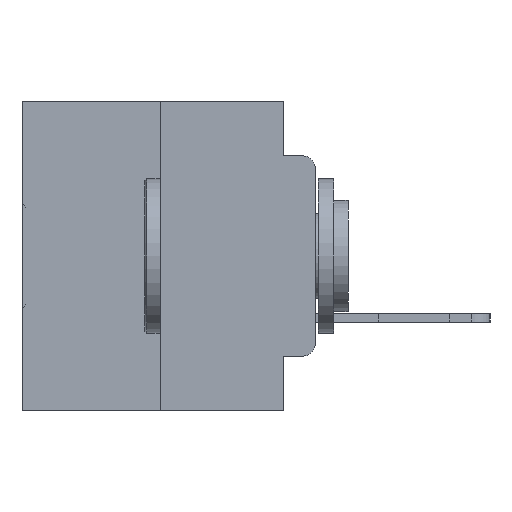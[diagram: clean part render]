
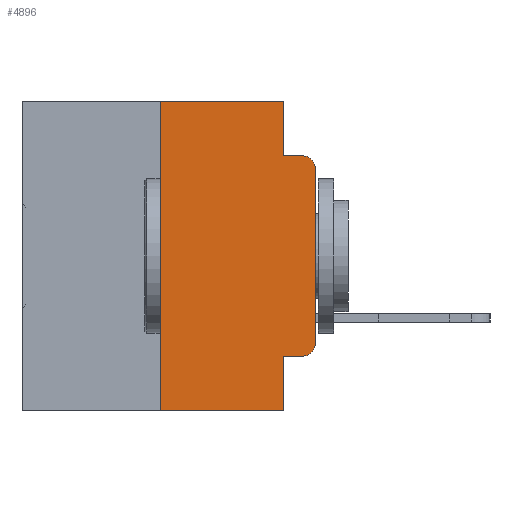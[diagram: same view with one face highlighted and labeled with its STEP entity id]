
A CAD part, left-side view. The second image highlights one B-rep face of the part: STEP entity #4896.
In plain terms, the highlighted planar face has unit normal (-1, 0, 0).
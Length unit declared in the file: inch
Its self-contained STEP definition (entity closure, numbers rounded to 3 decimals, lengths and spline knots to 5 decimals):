
#111 = DIRECTION ( 'NONE',  ( 1., 0., 0. ) ) ;
#134 = EDGE_CURVE ( 'NONE', #12930, #24687, #14888, .T. ) ;
#319 = VERTEX_POINT ( 'NONE', #17616 ) ;
#592 = LINE ( 'NONE', #30619, #20148 ) ;
#685 = EDGE_CURVE ( 'NONE', #12930, #2454, #32029, .T. ) ;
#907 = ORIENTED_EDGE ( 'NONE', *, *, #1544, .T. ) ;
#1107 = VERTEX_POINT ( 'NONE', #11351 ) ;
#1468 = DIRECTION ( 'NONE',  ( 0., -1., 0. ) ) ;
#1480 = VERTEX_POINT ( 'NONE', #30564 ) ;
#1495 = EDGE_CURVE ( 'NONE', #1683, #2454, #27915, .T. ) ;
#1544 = EDGE_CURVE ( 'NONE', #28971, #1480, #7253, .T. ) ;
#1683 = VERTEX_POINT ( 'NONE', #4377 ) ;
#1849 = CARTESIAN_POINT ( 'NONE',  ( 0., 0., -0.1085 ) ) ;
#1937 = DIRECTION ( 'NONE',  ( -1., 0., 0. ) ) ;
#1981 = CARTESIAN_POINT ( 'NONE',  ( 0., 0.02, -0.3915 ) ) ;
#2454 = VERTEX_POINT ( 'NONE', #27882 ) ;
#2876 = ORIENTED_EDGE ( 'NONE', *, *, #24950, .T. ) ;
#4190 = LINE ( 'NONE', #21783, #23527 ) ;
#4351 = ORIENTED_EDGE ( 'NONE', *, *, #9702, .F. ) ;
#4377 = CARTESIAN_POINT ( 'NONE',  ( 0., 0.051, -0.4115 ) ) ;
#4588 = VECTOR ( 'NONE', #20699, 39.37008 ) ;
#4867 = AXIS2_PLACEMENT_3D ( 'NONE', #1981, #1937, #8442 ) ;
#4896 = ADVANCED_FACE ( 'NONE', ( #6239 ), #30189, .F. ) ;
#5171 = AXIS2_PLACEMENT_3D ( 'NONE', #20436, #111, #18013 ) ;
#5403 = LINE ( 'NONE', #20583, #4588 ) ;
#6239 = FACE_OUTER_BOUND ( 'NONE', #18719, .T. ) ;
#6587 = ORIENTED_EDGE ( 'NONE', *, *, #7366, .F. ) ;
#7253 = CIRCLE ( 'NONE', #4867, 0.02 ) ;
#7366 = EDGE_CURVE ( 'NONE', #319, #1107, #592, .T. ) ;
#7780 = DIRECTION ( 'NONE',  ( 0., -1., 0. ) ) ;
#8157 = VECTOR ( 'NONE', #28744, 39.37008 ) ;
#8442 = DIRECTION ( 'NONE',  ( 0., 0., -1. ) ) ;
#9481 = CARTESIAN_POINT ( 'NONE',  ( 0., 0.02, -0.0885 ) ) ;
#9503 = EDGE_CURVE ( 'NONE', #1480, #29714, #4190, .T. ) ;
#9702 = EDGE_CURVE ( 'NONE', #1107, #24849, #5403, .T. ) ;
#10078 = ORIENTED_EDGE ( 'NONE', *, *, #28883, .F. ) ;
#11309 = ORIENTED_EDGE ( 'NONE', *, *, #9503, .T. ) ;
#11351 = CARTESIAN_POINT ( 'NONE',  ( 0., 0.051, -0.0885 ) ) ;
#11718 = ORIENTED_EDGE ( 'NONE', *, *, #134, .F. ) ;
#11906 = AXIS2_PLACEMENT_3D ( 'NONE', #15113, #32168, #17610 ) ;
#12418 = ORIENTED_EDGE ( 'NONE', *, *, #685, .T. ) ;
#12930 = VERTEX_POINT ( 'NONE', #28970 ) ;
#14179 = CARTESIAN_POINT ( 'NONE',  ( 0., 0.051, -0.4115 ) ) ;
#14397 = ORIENTED_EDGE ( 'NONE', *, *, #1495, .F. ) ;
#14888 = LINE ( 'NONE', #28805, #8157 ) ;
#15113 = CARTESIAN_POINT ( 'NONE',  ( 0., 0.02, -0.1085 ) ) ;
#17610 = DIRECTION ( 'NONE',  ( 0., 0., -1. ) ) ;
#17616 = CARTESIAN_POINT ( 'NONE',  ( 0., 0.051, 0. ) ) ;
#17891 = VECTOR ( 'NONE', #23906, 39.37008 ) ;
#18013 = DIRECTION ( 'NONE',  ( 0., 0., -1. ) ) ;
#18457 = DIRECTION ( 'NONE',  ( 0., 0., -1. ) ) ;
#18719 = EDGE_LOOP ( 'NONE', ( #11309, #2876, #4351, #6587, #10078, #11718, #12418, #14397, #23063, #907 ) ) ;
#19334 = VECTOR ( 'NONE', #1468, 39.37008 ) ;
#19455 = EDGE_CURVE ( 'NONE', #1683, #28971, #25876, .T. ) ;
#20148 = VECTOR ( 'NONE', #18457, 39.37008 ) ;
#20436 = CARTESIAN_POINT ( 'NONE',  ( 0., 0.473, 0. ) ) ;
#20583 = CARTESIAN_POINT ( 'NONE',  ( 0., 0.051, -0.0885 ) ) ;
#20699 = DIRECTION ( 'NONE',  ( 0., -1., 0. ) ) ;
#20827 = DIRECTION ( 'NONE',  ( 0., 0., -1. ) ) ;
#21142 = CARTESIAN_POINT ( 'NONE',  ( 0., 0.051, 0. ) ) ;
#21782 = CARTESIAN_POINT ( 'NONE',  ( 0., 0.02, -0.4115 ) ) ;
#21783 = CARTESIAN_POINT ( 'NONE',  ( 0., 0., 0. ) ) ;
#23063 = ORIENTED_EDGE ( 'NONE', *, *, #19455, .T. ) ;
#23527 = VECTOR ( 'NONE', #29104, 39.37008 ) ;
#23690 = CARTESIAN_POINT ( 'NONE',  ( 0., 0.25, 0. ) ) ;
#23906 = DIRECTION ( 'NONE',  ( 0., -1., 0. ) ) ;
#23916 = CARTESIAN_POINT ( 'NONE',  ( 0., 0.473, -0.5 ) ) ;
#24687 = VERTEX_POINT ( 'NONE', #23690 ) ;
#24849 = VERTEX_POINT ( 'NONE', #9481 ) ;
#24950 = EDGE_CURVE ( 'NONE', #29714, #24849, #29225, .T. ) ;
#25684 = VECTOR ( 'NONE', #7780, 39.37008 ) ;
#25876 = LINE ( 'NONE', #14179, #19334 ) ;
#26373 = CARTESIAN_POINT ( 'NONE',  ( 0., 0.473, 0. ) ) ;
#27146 = VECTOR ( 'NONE', #20827, 39.37008 ) ;
#27882 = CARTESIAN_POINT ( 'NONE',  ( 0., 0.051, -0.5 ) ) ;
#27915 = LINE ( 'NONE', #21142, #27146 ) ;
#28744 = DIRECTION ( 'NONE',  ( 0., 0., 1. ) ) ;
#28805 = CARTESIAN_POINT ( 'NONE',  ( 0., 0.25, 0. ) ) ;
#28883 = EDGE_CURVE ( 'NONE', #24687, #319, #30844, .T. ) ;
#28970 = CARTESIAN_POINT ( 'NONE',  ( 0., 0.25, -0.5 ) ) ;
#28971 = VERTEX_POINT ( 'NONE', #21782 ) ;
#29104 = DIRECTION ( 'NONE',  ( 0., 0., 1. ) ) ;
#29225 = CIRCLE ( 'NONE', #11906, 0.02 ) ;
#29714 = VERTEX_POINT ( 'NONE', #1849 ) ;
#30189 = PLANE ( 'NONE',  #5171 ) ;
#30564 = CARTESIAN_POINT ( 'NONE',  ( 0., 0., -0.3915 ) ) ;
#30619 = CARTESIAN_POINT ( 'NONE',  ( 0., 0.051, 0. ) ) ;
#30844 = LINE ( 'NONE', #26373, #17891 ) ;
#32029 = LINE ( 'NONE', #23916, #25684 ) ;
#32168 = DIRECTION ( 'NONE',  ( -1., 0., 0. ) ) ;
